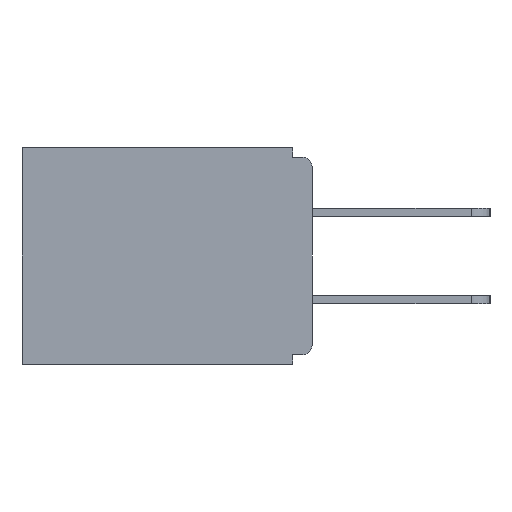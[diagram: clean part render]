
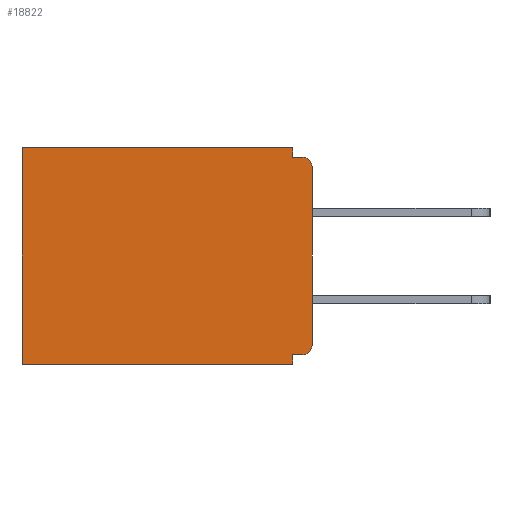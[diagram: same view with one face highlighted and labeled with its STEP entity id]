
A CAD part, left-side view. The second image highlights one B-rep face of the part: STEP entity #18822.
In plain terms, the highlighted planar face has unit normal (-1, 0, 0).
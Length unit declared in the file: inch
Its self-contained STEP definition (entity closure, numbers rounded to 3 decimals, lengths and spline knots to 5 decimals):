
#150 = DIRECTION ( 'NONE',  ( 1., 0., 0. ) ) ;
#229 = VERTEX_POINT ( 'NONE', #12263 ) ;
#264 = CARTESIAN_POINT ( 'NONE',  ( 0.298, 0., -0.313 ) ) ;
#857 = VECTOR ( 'NONE', #22866, 39.37008 ) ;
#1629 = VECTOR ( 'NONE', #20971, 39.37008 ) ;
#1831 = DIRECTION ( 'NONE',  ( -1., 0., 0. ) ) ;
#2459 = VERTEX_POINT ( 'NONE', #264 ) ;
#2917 = EDGE_CURVE ( 'NONE', #229, #4449, #24403, .T. ) ;
#3105 = CIRCLE ( 'NONE', #3135, 0.015 ) ;
#3135 = AXIS2_PLACEMENT_3D ( 'NONE', #3967, #1831, #19686 ) ;
#3585 = CARTESIAN_POINT ( 'NONE',  ( 0.298, 0.46, 0. ) ) ;
#3967 = CARTESIAN_POINT ( 'NONE',  ( 0.298, 0.015, -0.313 ) ) ;
#4037 = ORIENTED_EDGE ( 'NONE', *, *, #12610, .T. ) ;
#4055 = LINE ( 'NONE', #21953, #12413 ) ;
#4449 = VERTEX_POINT ( 'NONE', #3585 ) ;
#4826 = VECTOR ( 'NONE', #20259, 39.37008 ) ;
#4913 = VECTOR ( 'NONE', #19342, 39.37008 ) ;
#5849 = VECTOR ( 'NONE', #20042, 39.37008 ) ;
#6230 = LINE ( 'NONE', #13374, #4826 ) ;
#6260 = ORIENTED_EDGE ( 'NONE', *, *, #17642, .F. ) ;
#6856 = CARTESIAN_POINT ( 'NONE',  ( 0.298, 0.015, -0.03 ) ) ;
#6947 = ORIENTED_EDGE ( 'NONE', *, *, #17385, .F. ) ;
#7249 = CARTESIAN_POINT ( 'NONE',  ( 0.298, 0.46, -0.343 ) ) ;
#8738 = DIRECTION ( 'NONE',  ( 0., 1., 0. ) ) ;
#8876 = ORIENTED_EDGE ( 'NONE', *, *, #24305, .T. ) ;
#9058 = AXIS2_PLACEMENT_3D ( 'NONE', #22393, #150, #24720 ) ;
#9828 = CARTESIAN_POINT ( 'NONE',  ( 0.298, 0.031, -0.343 ) ) ;
#11537 = EDGE_CURVE ( 'NONE', #23527, #21469, #14093, .T. ) ;
#12212 = AXIS2_PLACEMENT_3D ( 'NONE', #6856, #13482, #13393 ) ;
#12259 = DIRECTION ( 'NONE',  ( 0., 0., -1. ) ) ;
#12263 = CARTESIAN_POINT ( 'NONE',  ( 0.298, 0.031, 0. ) ) ;
#12413 = VECTOR ( 'NONE', #8738, 39.37008 ) ;
#12610 = EDGE_CURVE ( 'NONE', #4449, #24664, #23220, .T. ) ;
#12980 = ORIENTED_EDGE ( 'NONE', *, *, #20882, .F. ) ;
#13168 = CARTESIAN_POINT ( 'NONE',  ( 0.298, 0.031, -0.015 ) ) ;
#13247 = CARTESIAN_POINT ( 'NONE',  ( 0.298, 0., -0.03 ) ) ;
#13374 = CARTESIAN_POINT ( 'NONE',  ( 0.298, 0., -0.015 ) ) ;
#13393 = DIRECTION ( 'NONE',  ( 0., 0., -1. ) ) ;
#13482 = DIRECTION ( 'NONE',  ( -1., 0., 0. ) ) ;
#13928 = VECTOR ( 'NONE', #12259, 39.37008 ) ;
#14093 = CIRCLE ( 'NONE', #12212, 0.015 ) ;
#14614 = CARTESIAN_POINT ( 'NONE',  ( 0.298, 0.015, -0.015 ) ) ;
#14945 = CARTESIAN_POINT ( 'NONE',  ( 0.298, 0.46, 0. ) ) ;
#15593 = PLANE ( 'NONE',  #9058 ) ;
#16157 = VERTEX_POINT ( 'NONE', #16194 ) ;
#16194 = CARTESIAN_POINT ( 'NONE',  ( 0.298, 0.031, -0.343 ) ) ;
#16338 = CARTESIAN_POINT ( 'NONE',  ( 0.298, 0.015, -0.328 ) ) ;
#16489 = ORIENTED_EDGE ( 'NONE', *, *, #11537, .T. ) ;
#17385 = EDGE_CURVE ( 'NONE', #16157, #24664, #18362, .T. ) ;
#17642 = EDGE_CURVE ( 'NONE', #23659, #20695, #4055, .T. ) ;
#17648 = CARTESIAN_POINT ( 'NONE',  ( 0.298, 0.031, -0.343 ) ) ;
#18362 = LINE ( 'NONE', #18881, #1629 ) ;
#18822 = ADVANCED_FACE ( 'NONE', ( #23335 ), #15593, .F. ) ;
#18881 = CARTESIAN_POINT ( 'NONE',  ( 0.298, 0., -0.343 ) ) ;
#19342 = DIRECTION ( 'NONE',  ( 0., 0., -1. ) ) ;
#19352 = ORIENTED_EDGE ( 'NONE', *, *, #25085, .F. ) ;
#19686 = DIRECTION ( 'NONE',  ( 0., 0., -1. ) ) ;
#19921 = ORIENTED_EDGE ( 'NONE', *, *, #2917, .T. ) ;
#19949 = LINE ( 'NONE', #26404, #4913 ) ;
#20042 = DIRECTION ( 'NONE',  ( 0., 1., 0. ) ) ;
#20153 = DIRECTION ( 'NONE',  ( 0., 0., -1. ) ) ;
#20259 = DIRECTION ( 'NONE',  ( 0., -1., 0. ) ) ;
#20406 = VECTOR ( 'NONE', #20153, 39.37008 ) ;
#20427 = ORIENTED_EDGE ( 'NONE', *, *, #22557, .F. ) ;
#20695 = VERTEX_POINT ( 'NONE', #28328 ) ;
#20845 = VERTEX_POINT ( 'NONE', #13168 ) ;
#20882 = EDGE_CURVE ( 'NONE', #20695, #16157, #28422, .T. ) ;
#20971 = DIRECTION ( 'NONE',  ( 0., 1., 0. ) ) ;
#21327 = LINE ( 'NONE', #9828, #13928 ) ;
#21469 = VERTEX_POINT ( 'NONE', #14614 ) ;
#21632 = ORIENTED_EDGE ( 'NONE', *, *, #23719, .F. ) ;
#21953 = CARTESIAN_POINT ( 'NONE',  ( 0.298, 0., -0.328 ) ) ;
#22393 = CARTESIAN_POINT ( 'NONE',  ( 0.298, 0., 0. ) ) ;
#22557 = EDGE_CURVE ( 'NONE', #23527, #2459, #19949, .T. ) ;
#22593 = EDGE_LOOP ( 'NONE', ( #16489, #19352, #21632, #19921, #4037, #6947, #12980, #6260, #8876, #20427 ) ) ;
#22866 = DIRECTION ( 'NONE',  ( 0., 0., -1. ) ) ;
#23220 = LINE ( 'NONE', #14945, #20406 ) ;
#23335 = FACE_OUTER_BOUND ( 'NONE', #22593, .T. ) ;
#23527 = VERTEX_POINT ( 'NONE', #13247 ) ;
#23659 = VERTEX_POINT ( 'NONE', #16338 ) ;
#23719 = EDGE_CURVE ( 'NONE', #229, #20845, #21327, .T. ) ;
#24305 = EDGE_CURVE ( 'NONE', #23659, #2459, #3105, .T. ) ;
#24403 = LINE ( 'NONE', #28527, #5849 ) ;
#24664 = VERTEX_POINT ( 'NONE', #7249 ) ;
#24720 = DIRECTION ( 'NONE',  ( 0., 0., -1. ) ) ;
#25085 = EDGE_CURVE ( 'NONE', #20845, #21469, #6230, .T. ) ;
#26404 = CARTESIAN_POINT ( 'NONE',  ( 0.298, 0., 0. ) ) ;
#28328 = CARTESIAN_POINT ( 'NONE',  ( 0.298, 0.031, -0.328 ) ) ;
#28422 = LINE ( 'NONE', #17648, #857 ) ;
#28527 = CARTESIAN_POINT ( 'NONE',  ( 0.298, 0., 0. ) ) ;
